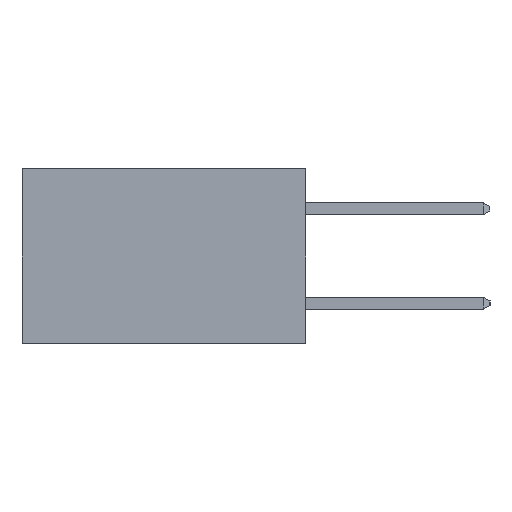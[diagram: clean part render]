
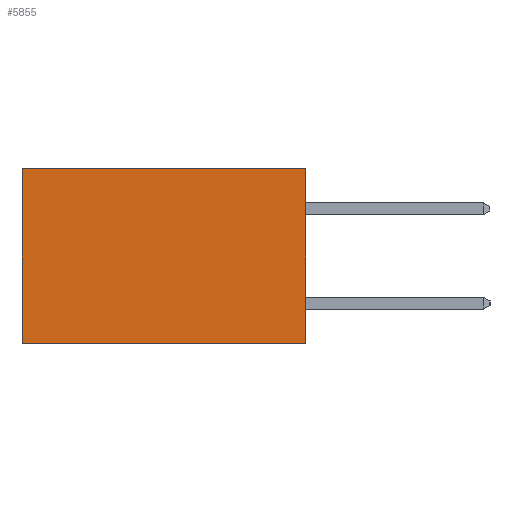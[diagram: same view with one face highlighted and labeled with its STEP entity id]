
A CAD part, left-side view. The second image highlights one B-rep face of the part: STEP entity #5855.
In plain terms, the highlighted planar face has unit normal (-1, 0, 0).
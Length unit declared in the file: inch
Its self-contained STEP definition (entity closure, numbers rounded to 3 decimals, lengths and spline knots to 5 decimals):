
#575 = CARTESIAN_POINT ( 'NONE',  ( 0.2615, 0., 0. ) ) ;
#1270 = CARTESIAN_POINT ( 'NONE',  ( 0.2615, 0., 0. ) ) ;
#1599 = AXIS2_PLACEMENT_3D ( 'NONE', #16220, #3161, #10948 ) ;
#1872 = CARTESIAN_POINT ( 'NONE',  ( 0.2615, 0.6, 0. ) ) ;
#1902 = VERTEX_POINT ( 'NONE', #1270 ) ;
#1982 = VERTEX_POINT ( 'NONE', #19670 ) ;
#3052 = CARTESIAN_POINT ( 'NONE',  ( 0.2615, 0., -0.37 ) ) ;
#3161 = DIRECTION ( 'NONE',  ( 1., 0., 0. ) ) ;
#3288 = ORIENTED_EDGE ( 'NONE', *, *, #16619, .F. ) ;
#3870 = CARTESIAN_POINT ( 'NONE',  ( 0.2615, 0.6, -0.37 ) ) ;
#5019 = DIRECTION ( 'NONE',  ( 0., 0., -1. ) ) ;
#5037 = LINE ( 'NONE', #3052, #18232 ) ;
#5302 = LINE ( 'NONE', #16827, #17513 ) ;
#5533 = VECTOR ( 'NONE', #5019, 39.37008 ) ;
#5855 = ADVANCED_FACE ( 'NONE', ( #15785 ), #11574, .F. ) ;
#6665 = EDGE_LOOP ( 'NONE', ( #18339, #14390, #3288, #15504 ) ) ;
#8270 = EDGE_CURVE ( 'NONE', #1902, #19893, #9468, .T. ) ;
#9468 = LINE ( 'NONE', #575, #17416 ) ;
#10250 = DIRECTION ( 'NONE',  ( 0., 1., 0. ) ) ;
#10948 = DIRECTION ( 'NONE',  ( 0., 0., -1. ) ) ;
#11574 = PLANE ( 'NONE',  #1599 ) ;
#12525 = VERTEX_POINT ( 'NONE', #3870 ) ;
#12951 = CARTESIAN_POINT ( 'NONE',  ( 0.2615, 0.6, -0.37 ) ) ;
#13713 = EDGE_CURVE ( 'NONE', #19893, #12525, #14538, .T. ) ;
#14234 = DIRECTION ( 'NONE',  ( 0., 1., 0. ) ) ;
#14390 = ORIENTED_EDGE ( 'NONE', *, *, #16844, .F. ) ;
#14538 = LINE ( 'NONE', #12951, #5533 ) ;
#15504 = ORIENTED_EDGE ( 'NONE', *, *, #8270, .T. ) ;
#15785 = FACE_OUTER_BOUND ( 'NONE', #6665, .T. ) ;
#16220 = CARTESIAN_POINT ( 'NONE',  ( 0.2615, 0., -0.37 ) ) ;
#16619 = EDGE_CURVE ( 'NONE', #1902, #1982, #5302, .T. ) ;
#16827 = CARTESIAN_POINT ( 'NONE',  ( 0.2615, 0., -0.37 ) ) ;
#16844 = EDGE_CURVE ( 'NONE', #1982, #12525, #5037, .T. ) ;
#17416 = VECTOR ( 'NONE', #10250, 39.37008 ) ;
#17513 = VECTOR ( 'NONE', #18373, 39.37008 ) ;
#18232 = VECTOR ( 'NONE', #14234, 39.37008 ) ;
#18339 = ORIENTED_EDGE ( 'NONE', *, *, #13713, .T. ) ;
#18373 = DIRECTION ( 'NONE',  ( 0., 0., -1. ) ) ;
#19670 = CARTESIAN_POINT ( 'NONE',  ( 0.2615, 0., -0.37 ) ) ;
#19893 = VERTEX_POINT ( 'NONE', #1872 ) ;
